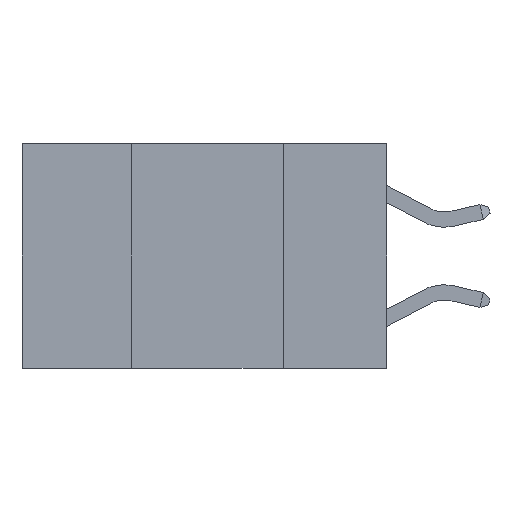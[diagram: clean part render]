
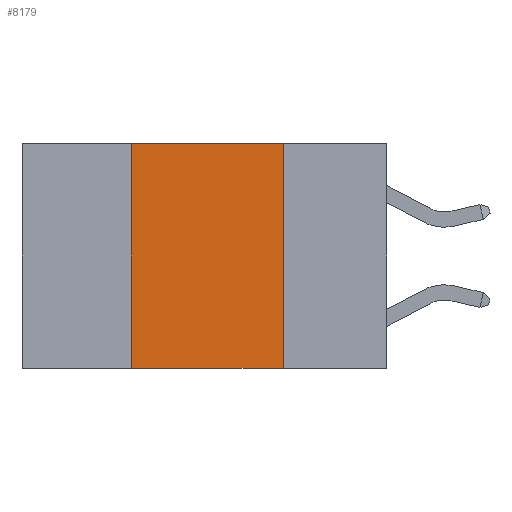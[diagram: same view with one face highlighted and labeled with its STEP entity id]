
A CAD part, left-side view. The second image highlights one B-rep face of the part: STEP entity #8179.
In plain terms, the highlighted planar face has unit normal (-1, 0, 0).
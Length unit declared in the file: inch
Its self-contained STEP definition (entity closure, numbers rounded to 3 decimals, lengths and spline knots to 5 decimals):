
#489 = VECTOR ( 'NONE', #3273, 39.37008 ) ;
#1528 = CARTESIAN_POINT ( 'NONE',  ( 0., 0.42, 0. ) ) ;
#1560 = VECTOR ( 'NONE', #3178, 39.37008 ) ;
#2579 = DIRECTION ( 'NONE',  ( 0., 0., -1. ) ) ;
#3178 = DIRECTION ( 'NONE',  ( 0., 0., 1. ) ) ;
#3273 = DIRECTION ( 'NONE',  ( 0., 0., -1. ) ) ;
#4078 = VECTOR ( 'NONE', #6585, 39.37008 ) ;
#4241 = PLANE ( 'NONE',  #15341 ) ;
#5328 = VERTEX_POINT ( 'NONE', #13648 ) ;
#6585 = DIRECTION ( 'NONE',  ( 0., -1., 0. ) ) ;
#8179 = ADVANCED_FACE ( 'NONE', ( #19887 ), #4241, .F. ) ;
#8510 = CARTESIAN_POINT ( 'NONE',  ( 0., 0.42, -0.37 ) ) ;
#10017 = CARTESIAN_POINT ( 'NONE',  ( 0., 0.17, 0. ) ) ;
#10126 = LINE ( 'NONE', #16756, #489 ) ;
#10172 = LINE ( 'NONE', #18606, #18471 ) ;
#10360 = EDGE_CURVE ( 'NONE', #5328, #15022, #10172, .T. ) ;
#10869 = VERTEX_POINT ( 'NONE', #11627 ) ;
#11060 = CARTESIAN_POINT ( 'NONE',  ( 0., 0.6, 0. ) ) ;
#11076 = VERTEX_POINT ( 'NONE', #8510 ) ;
#11627 = CARTESIAN_POINT ( 'NONE',  ( 0., 0.17, -0.37 ) ) ;
#12416 = EDGE_CURVE ( 'NONE', #11076, #5328, #15574, .T. ) ;
#12676 = ORIENTED_EDGE ( 'NONE', *, *, #18013, .F. ) ;
#12714 = DIRECTION ( 'NONE',  ( 1., 0., 0. ) ) ;
#13579 = LINE ( 'NONE', #14930, #4078 ) ;
#13648 = CARTESIAN_POINT ( 'NONE',  ( 0., 0.42, 0. ) ) ;
#14930 = CARTESIAN_POINT ( 'NONE',  ( 0., 0.6, -0.37 ) ) ;
#15022 = VERTEX_POINT ( 'NONE', #10017 ) ;
#15341 = AXIS2_PLACEMENT_3D ( 'NONE', #11060, #12714, #2579 ) ;
#15574 = LINE ( 'NONE', #1528, #1560 ) ;
#15779 = EDGE_CURVE ( 'NONE', #11076, #10869, #13579, .T. ) ;
#16298 = EDGE_LOOP ( 'NONE', ( #12676, #21439, #20673, #17465 ) ) ;
#16756 = CARTESIAN_POINT ( 'NONE',  ( 0., 0.17, 0. ) ) ;
#17465 = ORIENTED_EDGE ( 'NONE', *, *, #15779, .T. ) ;
#18013 = EDGE_CURVE ( 'NONE', #15022, #10869, #10126, .T. ) ;
#18471 = VECTOR ( 'NONE', #20268, 39.37008 ) ;
#18606 = CARTESIAN_POINT ( 'NONE',  ( 0., 0.6, 0. ) ) ;
#19887 = FACE_OUTER_BOUND ( 'NONE', #16298, .T. ) ;
#20268 = DIRECTION ( 'NONE',  ( 0., -1., 0. ) ) ;
#20673 = ORIENTED_EDGE ( 'NONE', *, *, #12416, .F. ) ;
#21439 = ORIENTED_EDGE ( 'NONE', *, *, #10360, .F. ) ;
